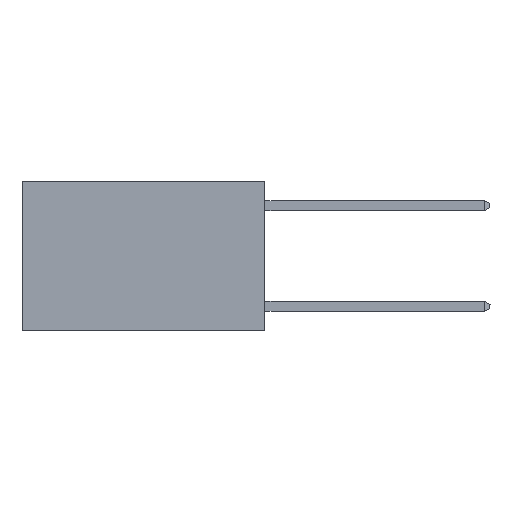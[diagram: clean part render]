
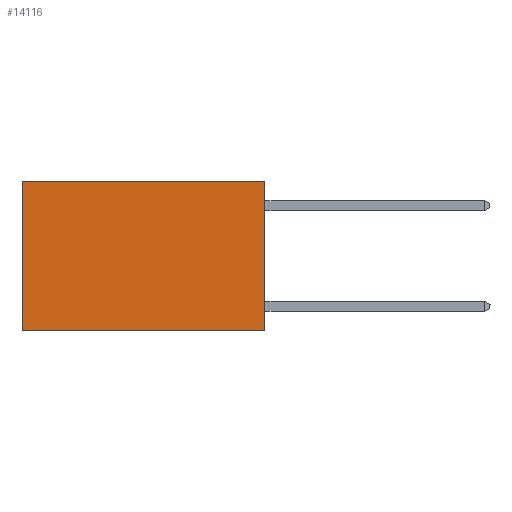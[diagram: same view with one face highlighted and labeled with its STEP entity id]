
A CAD part, left-side view. The second image highlights one B-rep face of the part: STEP entity #14116.
In plain terms, the highlighted planar face has unit normal (-1, 0, 0).
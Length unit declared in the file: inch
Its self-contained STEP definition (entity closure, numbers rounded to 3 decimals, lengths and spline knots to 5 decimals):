
#1324 = VERTEX_POINT ( 'NONE', #15924 ) ;
#1853 = CARTESIAN_POINT ( 'NONE',  ( 0.2625, 0.6, -0.37 ) ) ;
#1897 = PLANE ( 'NONE',  #12026 ) ;
#2011 = CARTESIAN_POINT ( 'NONE',  ( 0.2625, 0., -0.37 ) ) ;
#2719 = VECTOR ( 'NONE', #6810, 39.37008 ) ;
#3304 = CARTESIAN_POINT ( 'NONE',  ( 0.2625, 0., 0. ) ) ;
#3456 = VERTEX_POINT ( 'NONE', #15319 ) ;
#4043 = VECTOR ( 'NONE', #12350, 39.37008 ) ;
#4092 = ORIENTED_EDGE ( 'NONE', *, *, #11463, .F. ) ;
#4097 = EDGE_CURVE ( 'NONE', #1324, #4831, #15582, .T. ) ;
#4414 = CARTESIAN_POINT ( 'NONE',  ( 0.2625, 0., 0. ) ) ;
#4472 = LINE ( 'NONE', #15229, #4043 ) ;
#4702 = DIRECTION ( 'NONE',  ( 1., 0., 0. ) ) ;
#4748 = LINE ( 'NONE', #4414, #8024 ) ;
#4831 = VERTEX_POINT ( 'NONE', #1853 ) ;
#4914 = CARTESIAN_POINT ( 'NONE',  ( 0.2625, 0.6, 0. ) ) ;
#5413 = CARTESIAN_POINT ( 'NONE',  ( 0.2625, 0., 0. ) ) ;
#6810 = DIRECTION ( 'NONE',  ( 0., 0., -1. ) ) ;
#6913 = EDGE_CURVE ( 'NONE', #3456, #1324, #4748, .T. ) ;
#8024 = VECTOR ( 'NONE', #8649, 39.37008 ) ;
#8345 = VECTOR ( 'NONE', #10581, 39.37008 ) ;
#8649 = DIRECTION ( 'NONE',  ( 0., 1., 0. ) ) ;
#10581 = DIRECTION ( 'NONE',  ( 0., 0., -1. ) ) ;
#10701 = ORIENTED_EDGE ( 'NONE', *, *, #4097, .T. ) ;
#11463 = EDGE_CURVE ( 'NONE', #3456, #11829, #14110, .T. ) ;
#11596 = ORIENTED_EDGE ( 'NONE', *, *, #6913, .T. ) ;
#11829 = VERTEX_POINT ( 'NONE', #2011 ) ;
#12026 = AXIS2_PLACEMENT_3D ( 'NONE', #3304, #4702, #14720 ) ;
#12350 = DIRECTION ( 'NONE',  ( 0., 1., 0. ) ) ;
#14110 = LINE ( 'NONE', #5413, #2719 ) ;
#14116 = ADVANCED_FACE ( 'NONE', ( #14205 ), #1897, .F. ) ;
#14205 = FACE_OUTER_BOUND ( 'NONE', #17517, .T. ) ;
#14720 = DIRECTION ( 'NONE',  ( 0., 0., -1. ) ) ;
#15229 = CARTESIAN_POINT ( 'NONE',  ( 0.2625, 0., -0.37 ) ) ;
#15319 = CARTESIAN_POINT ( 'NONE',  ( 0.2625, 0., 0. ) ) ;
#15551 = EDGE_CURVE ( 'NONE', #11829, #4831, #4472, .T. ) ;
#15582 = LINE ( 'NONE', #4914, #8345 ) ;
#15924 = CARTESIAN_POINT ( 'NONE',  ( 0.2625, 0.6, 0. ) ) ;
#17517 = EDGE_LOOP ( 'NONE', ( #10701, #18323, #4092, #11596 ) ) ;
#18323 = ORIENTED_EDGE ( 'NONE', *, *, #15551, .F. ) ;
